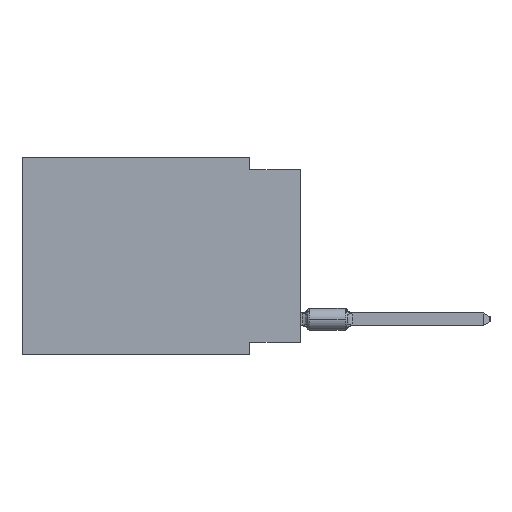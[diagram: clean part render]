
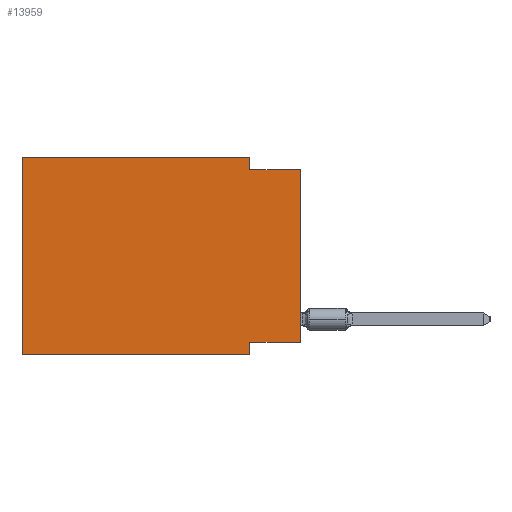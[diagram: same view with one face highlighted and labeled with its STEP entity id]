
A CAD part, left-side view. The second image highlights one B-rep face of the part: STEP entity #13959.
In plain terms, the highlighted planar face has unit normal (-1, 0, 0).
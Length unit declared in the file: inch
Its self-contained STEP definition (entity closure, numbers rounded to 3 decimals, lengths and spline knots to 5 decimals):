
#936 = VECTOR ( 'NONE', #20952, 39.37008 ) ;
#1767 = EDGE_LOOP ( 'NONE', ( #47425, #14005, #16214, #3731, #4799, #26347, #43715, #31089 ) ) ;
#3117 = CARTESIAN_POINT ( 'NONE',  ( 0., 0.55, 0. ) ) ;
#3570 = CARTESIAN_POINT ( 'NONE',  ( 0., 0.1, -0.39 ) ) ;
#3731 = ORIENTED_EDGE ( 'NONE', *, *, #5598, .F. ) ;
#3821 = LINE ( 'NONE', #37578, #36672 ) ;
#3987 = VECTOR ( 'NONE', #39734, 39.37008 ) ;
#4799 = ORIENTED_EDGE ( 'NONE', *, *, #37867, .F. ) ;
#5156 = CARTESIAN_POINT ( 'NONE',  ( 0., 0.1, 0. ) ) ;
#5266 = VECTOR ( 'NONE', #18623, 39.37008 ) ;
#5598 = EDGE_CURVE ( 'NONE', #37353, #13054, #35021, .T. ) ;
#5637 = DIRECTION ( 'NONE',  ( 0., -1., 0. ) ) ;
#6155 = VERTEX_POINT ( 'NONE', #3570 ) ;
#7083 = EDGE_CURVE ( 'NONE', #53670, #6155, #37477, .T. ) ;
#7742 = CARTESIAN_POINT ( 'NONE',  ( 0., 0., -0.025 ) ) ;
#9149 = DIRECTION ( 'NONE',  ( 0., 0., 1. ) ) ;
#10544 = CARTESIAN_POINT ( 'NONE',  ( 0., 0.1, -0.365 ) ) ;
#11747 = LINE ( 'NONE', #5156, #936 ) ;
#13054 = VERTEX_POINT ( 'NONE', #45495 ) ;
#13959 = ADVANCED_FACE ( 'NONE', ( #16142 ), #32506, .F. ) ;
#14005 = ORIENTED_EDGE ( 'NONE', *, *, #44812, .F. ) ;
#15163 = LINE ( 'NONE', #43272, #3987 ) ;
#16043 = CARTESIAN_POINT ( 'NONE',  ( 0., 0.1, -0.025 ) ) ;
#16142 = FACE_OUTER_BOUND ( 'NONE', #1767, .T. ) ;
#16214 = ORIENTED_EDGE ( 'NONE', *, *, #39763, .F. ) ;
#16484 = DIRECTION ( 'NONE',  ( 0., 0., -1. ) ) ;
#17139 = DIRECTION ( 'NONE',  ( 0., 1., 0. ) ) ;
#17783 = VECTOR ( 'NONE', #48075, 39.37008 ) ;
#18623 = DIRECTION ( 'NONE',  ( 0., 0., 1. ) ) ;
#20615 = VERTEX_POINT ( 'NONE', #16043 ) ;
#20952 = DIRECTION ( 'NONE',  ( 0., 0., -1. ) ) ;
#22086 = VECTOR ( 'NONE', #16484, 39.37008 ) ;
#23006 = LINE ( 'NONE', #3117, #5266 ) ;
#26347 = ORIENTED_EDGE ( 'NONE', *, *, #46002, .T. ) ;
#26624 = CARTESIAN_POINT ( 'NONE',  ( 0., 0.55, 0. ) ) ;
#27158 = CARTESIAN_POINT ( 'NONE',  ( 0., 0., -0.365 ) ) ;
#27219 = VECTOR ( 'NONE', #9149, 39.37008 ) ;
#27696 = VECTOR ( 'NONE', #5637, 39.37008 ) ;
#28166 = DIRECTION ( 'NONE',  ( 0., 0., -1. ) ) ;
#28248 = VERTEX_POINT ( 'NONE', #27158 ) ;
#30037 = VERTEX_POINT ( 'NONE', #46138 ) ;
#31089 = ORIENTED_EDGE ( 'NONE', *, *, #41308, .F. ) ;
#32506 = PLANE ( 'NONE',  #50880 ) ;
#33303 = CARTESIAN_POINT ( 'NONE',  ( 0., 0.55, 0. ) ) ;
#33936 = CARTESIAN_POINT ( 'NONE',  ( 0., 0., 0. ) ) ;
#35021 = LINE ( 'NONE', #42951, #27696 ) ;
#36672 = VECTOR ( 'NONE', #17139, 39.37008 ) ;
#37353 = VERTEX_POINT ( 'NONE', #26624 ) ;
#37477 = LINE ( 'NONE', #41300, #22086 ) ;
#37578 = CARTESIAN_POINT ( 'NONE',  ( 0., 0., -0.365 ) ) ;
#37867 = EDGE_CURVE ( 'NONE', #30037, #37353, #23006, .T. ) ;
#39734 = DIRECTION ( 'NONE',  ( 0., -1., 0. ) ) ;
#39763 = EDGE_CURVE ( 'NONE', #13054, #20615, #11747, .T. ) ;
#40524 = CARTESIAN_POINT ( 'NONE',  ( 0., 0., -0.025 ) ) ;
#41300 = CARTESIAN_POINT ( 'NONE',  ( 0., 0.1, -0.39 ) ) ;
#41308 = EDGE_CURVE ( 'NONE', #28248, #53670, #3821, .T. ) ;
#42554 = EDGE_CURVE ( 'NONE', #28248, #48003, #51102, .T. ) ;
#42951 = CARTESIAN_POINT ( 'NONE',  ( 0., 0.55, 0. ) ) ;
#43272 = CARTESIAN_POINT ( 'NONE',  ( 0., 0.55, -0.39 ) ) ;
#43715 = ORIENTED_EDGE ( 'NONE', *, *, #7083, .F. ) ;
#44812 = EDGE_CURVE ( 'NONE', #20615, #48003, #52713, .T. ) ;
#45495 = CARTESIAN_POINT ( 'NONE',  ( 0., 0.1, 0. ) ) ;
#45572 = DIRECTION ( 'NONE',  ( 1., 0., 0. ) ) ;
#46002 = EDGE_CURVE ( 'NONE', #30037, #6155, #15163, .T. ) ;
#46138 = CARTESIAN_POINT ( 'NONE',  ( 0., 0.55, -0.39 ) ) ;
#47425 = ORIENTED_EDGE ( 'NONE', *, *, #42554, .T. ) ;
#48003 = VERTEX_POINT ( 'NONE', #40524 ) ;
#48075 = DIRECTION ( 'NONE',  ( 0., -1., 0. ) ) ;
#50880 = AXIS2_PLACEMENT_3D ( 'NONE', #33303, #45572, #28166 ) ;
#51102 = LINE ( 'NONE', #33936, #27219 ) ;
#52713 = LINE ( 'NONE', #7742, #17783 ) ;
#53670 = VERTEX_POINT ( 'NONE', #10544 ) ;
